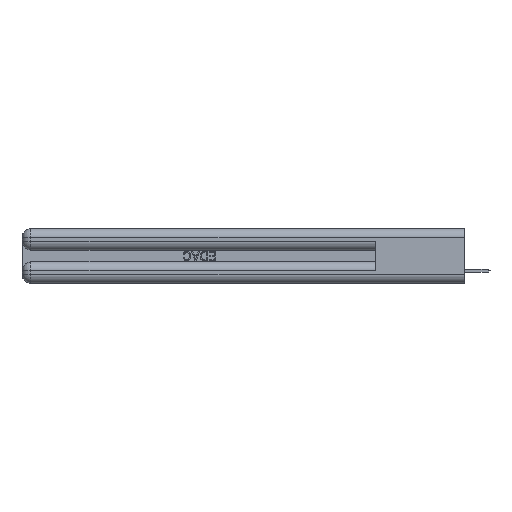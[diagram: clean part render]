
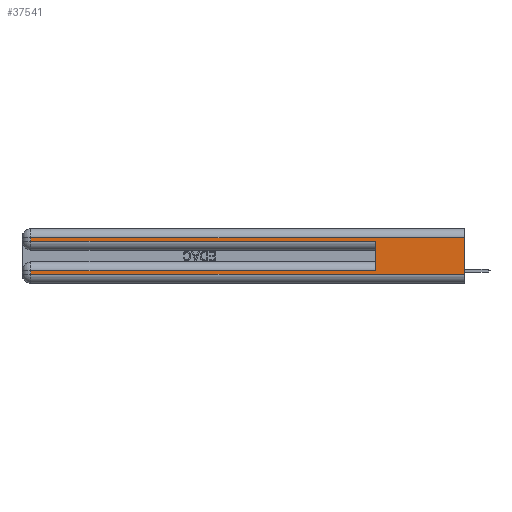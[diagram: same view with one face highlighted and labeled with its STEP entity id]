
A CAD part, left-side view. The second image highlights one B-rep face of the part: STEP entity #37541.
In plain terms, the highlighted planar face has unit normal (-1, 0, 0).
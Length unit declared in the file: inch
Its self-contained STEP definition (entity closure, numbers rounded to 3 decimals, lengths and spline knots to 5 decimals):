
#1026 = LINE ( 'NONE', #24885, #6124 ) ;
#2087 = DIRECTION ( 'NONE',  ( 0., 0., 1. ) ) ;
#3279 = CARTESIAN_POINT ( 'NONE',  ( 0., 0.6, 0.285 ) ) ;
#3573 = LINE ( 'NONE', #20788, #46600 ) ;
#3835 = CARTESIAN_POINT ( 'NONE',  ( 0., 0., 0.37 ) ) ;
#6033 = ORIENTED_EDGE ( 'NONE', *, *, #33790, .F. ) ;
#6087 = EDGE_CURVE ( 'NONE', #31047, #28657, #1026, .T. ) ;
#6124 = VECTOR ( 'NONE', #21120, 39.37008 ) ;
#7973 = CARTESIAN_POINT ( 'NONE',  ( 0., 0., 0.285 ) ) ;
#8372 = VERTEX_POINT ( 'NONE', #50699 ) ;
#8869 = AXIS2_PLACEMENT_3D ( 'NONE', #17079, #45350, #24743 ) ;
#9801 = CARTESIAN_POINT ( 'NONE',  ( 0., 2.94, 0.06 ) ) ;
#10603 = ORIENTED_EDGE ( 'NONE', *, *, #21082, .F. ) ;
#11244 = LINE ( 'NONE', #3835, #52326 ) ;
#12028 = DIRECTION ( 'NONE',  ( 0., 0., -1. ) ) ;
#12400 = DIRECTION ( 'NONE',  ( 0., -1., 0. ) ) ;
#17079 = CARTESIAN_POINT ( 'NONE',  ( 0., 0., 0.37 ) ) ;
#17448 = ORIENTED_EDGE ( 'NONE', *, *, #18445, .T. ) ;
#17594 = CARTESIAN_POINT ( 'NONE',  ( 0., 2.94, 0.085 ) ) ;
#18445 = EDGE_CURVE ( 'NONE', #24763, #30461, #20870, .T. ) ;
#19570 = CARTESIAN_POINT ( 'NONE',  ( 0., 2.94, 0.37 ) ) ;
#20402 = FACE_OUTER_BOUND ( 'NONE', #49433, .T. ) ;
#20788 = CARTESIAN_POINT ( 'NONE',  ( 0., 0.6, 0.145 ) ) ;
#20870 = LINE ( 'NONE', #42822, #36659 ) ;
#21082 = EDGE_CURVE ( 'NONE', #31047, #30461, #11244, .T. ) ;
#21120 = DIRECTION ( 'NONE',  ( 0., 1., 0. ) ) ;
#21394 = LINE ( 'NONE', #19570, #52380 ) ;
#23393 = VECTOR ( 'NONE', #46521, 39.37008 ) ;
#23997 = CARTESIAN_POINT ( 'NONE',  ( 0., 0.6, 0.085 ) ) ;
#24743 = DIRECTION ( 'NONE',  ( 0., 0., -1. ) ) ;
#24763 = VERTEX_POINT ( 'NONE', #9801 ) ;
#24885 = CARTESIAN_POINT ( 'NONE',  ( 0., 0., 0.31 ) ) ;
#26878 = EDGE_CURVE ( 'NONE', #28657, #8372, #44794, .T. ) ;
#27339 = DIRECTION ( 'NONE',  ( 0., 0., -1. ) ) ;
#28657 = VERTEX_POINT ( 'NONE', #51488 ) ;
#29224 = EDGE_CURVE ( 'NONE', #46435, #36176, #40939, .T. ) ;
#30426 = ORIENTED_EDGE ( 'NONE', *, *, #6087, .T. ) ;
#30461 = VERTEX_POINT ( 'NONE', #32204 ) ;
#30817 = VECTOR ( 'NONE', #39735, 39.37008 ) ;
#31047 = VERTEX_POINT ( 'NONE', #49004 ) ;
#32204 = CARTESIAN_POINT ( 'NONE',  ( 0., 0., 0.06 ) ) ;
#32759 = ORIENTED_EDGE ( 'NONE', *, *, #48144, .T. ) ;
#33790 = EDGE_CURVE ( 'NONE', #46435, #50748, #3573, .T. ) ;
#36176 = VERTEX_POINT ( 'NONE', #17594 ) ;
#36659 = VECTOR ( 'NONE', #43335, 39.37008 ) ;
#37108 = VECTOR ( 'NONE', #12400, 39.37008 ) ;
#37541 = ADVANCED_FACE ( 'NONE', ( #20402 ), #45169, .F. ) ;
#39735 = DIRECTION ( 'NONE',  ( 0., 1., 0. ) ) ;
#40576 = ORIENTED_EDGE ( 'NONE', *, *, #43338, .T. ) ;
#40939 = LINE ( 'NONE', #43289, #30817 ) ;
#42511 = CARTESIAN_POINT ( 'NONE',  ( 0., 2.94, 0.37 ) ) ;
#42653 = ORIENTED_EDGE ( 'NONE', *, *, #26878, .T. ) ;
#42822 = CARTESIAN_POINT ( 'NONE',  ( 0., 0., 0.06 ) ) ;
#43289 = CARTESIAN_POINT ( 'NONE',  ( 0., 0., 0.085 ) ) ;
#43335 = DIRECTION ( 'NONE',  ( 0., -1., 0. ) ) ;
#43338 = EDGE_CURVE ( 'NONE', #8372, #50748, #51037, .T. ) ;
#44794 = LINE ( 'NONE', #42511, #23393 ) ;
#45169 = PLANE ( 'NONE',  #8869 ) ;
#45350 = DIRECTION ( 'NONE',  ( 1., 0., 0. ) ) ;
#46435 = VERTEX_POINT ( 'NONE', #23997 ) ;
#46521 = DIRECTION ( 'NONE',  ( 0., 0., -1. ) ) ;
#46600 = VECTOR ( 'NONE', #2087, 39.37008 ) ;
#48144 = EDGE_CURVE ( 'NONE', #36176, #24763, #21394, .T. ) ;
#49004 = CARTESIAN_POINT ( 'NONE',  ( 0., 0., 0.31 ) ) ;
#49433 = EDGE_LOOP ( 'NONE', ( #10603, #30426, #42653, #40576, #6033, #51772, #32759, #17448 ) ) ;
#50699 = CARTESIAN_POINT ( 'NONE',  ( 0., 2.94, 0.285 ) ) ;
#50748 = VERTEX_POINT ( 'NONE', #3279 ) ;
#51037 = LINE ( 'NONE', #7973, #37108 ) ;
#51488 = CARTESIAN_POINT ( 'NONE',  ( 0., 2.94, 0.31 ) ) ;
#51772 = ORIENTED_EDGE ( 'NONE', *, *, #29224, .T. ) ;
#52326 = VECTOR ( 'NONE', #12028, 39.37008 ) ;
#52380 = VECTOR ( 'NONE', #27339, 39.37008 ) ;
